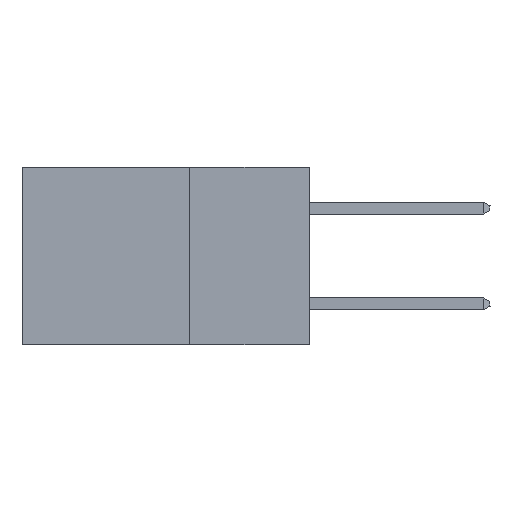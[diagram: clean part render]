
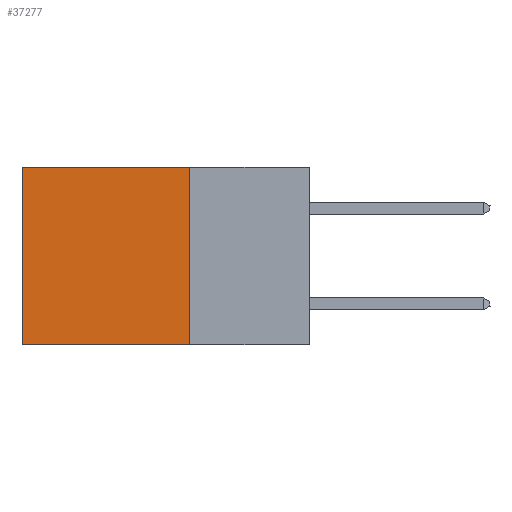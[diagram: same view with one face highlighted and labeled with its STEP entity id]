
A CAD part, left-side view. The second image highlights one B-rep face of the part: STEP entity #37277.
In plain terms, the highlighted planar face has unit normal (-1, 0, 0).
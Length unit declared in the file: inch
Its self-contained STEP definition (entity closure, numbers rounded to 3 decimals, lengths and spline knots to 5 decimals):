
#478 = VECTOR ( 'NONE', #3477, 39.37008 ) ;
#698 = DIRECTION ( 'NONE',  ( 0., 0., -1. ) ) ;
#1804 = VERTEX_POINT ( 'NONE', #7959 ) ;
#3477 = DIRECTION ( 'NONE',  ( 0., 0., -1. ) ) ;
#5650 = LINE ( 'NONE', #15733, #6616 ) ;
#5654 = CARTESIAN_POINT ( 'NONE',  ( 0.2875, 0.6, 0. ) ) ;
#6616 = VECTOR ( 'NONE', #9685, 39.37008 ) ;
#7645 = VECTOR ( 'NONE', #698, 39.37008 ) ;
#7959 = CARTESIAN_POINT ( 'NONE',  ( 0.2875, 0.25, -0.37 ) ) ;
#8752 = LINE ( 'NONE', #30887, #478 ) ;
#8834 = CARTESIAN_POINT ( 'NONE',  ( 0.2875, 0.6, -0.37 ) ) ;
#8905 = ORIENTED_EDGE ( 'NONE', *, *, #13573, .F. ) ;
#9685 = DIRECTION ( 'NONE',  ( 0., 1., 0. ) ) ;
#10686 = ORIENTED_EDGE ( 'NONE', *, *, #37093, .F. ) ;
#11004 = EDGE_CURVE ( 'NONE', #24900, #12206, #8752, .T. ) ;
#12206 = VERTEX_POINT ( 'NONE', #8834 ) ;
#12350 = VECTOR ( 'NONE', #13617, 39.37008 ) ;
#13573 = EDGE_CURVE ( 'NONE', #31010, #1804, #31904, .T. ) ;
#13617 = DIRECTION ( 'NONE',  ( 0., 1., 0. ) ) ;
#14423 = PLANE ( 'NONE',  #36116 ) ;
#15595 = EDGE_CURVE ( 'NONE', #31010, #24900, #5650, .T. ) ;
#15733 = CARTESIAN_POINT ( 'NONE',  ( 0.2875, 0.25, 0. ) ) ;
#16137 = CARTESIAN_POINT ( 'NONE',  ( 0.2875, 0.25, 0. ) ) ;
#20641 = DIRECTION ( 'NONE',  ( 0., 0., -1. ) ) ;
#21948 = FACE_OUTER_BOUND ( 'NONE', #30113, .T. ) ;
#23592 = CARTESIAN_POINT ( 'NONE',  ( 0.2875, 0.25, 0. ) ) ;
#24900 = VERTEX_POINT ( 'NONE', #5654 ) ;
#26756 = ORIENTED_EDGE ( 'NONE', *, *, #11004, .T. ) ;
#28531 = LINE ( 'NONE', #28797, #12350 ) ;
#28797 = CARTESIAN_POINT ( 'NONE',  ( 0.2875, 0.25, -0.37 ) ) ;
#30113 = EDGE_LOOP ( 'NONE', ( #26756, #10686, #8905, #38354 ) ) ;
#30887 = CARTESIAN_POINT ( 'NONE',  ( 0.2875, 0.6, 0. ) ) ;
#31010 = VERTEX_POINT ( 'NONE', #23592 ) ;
#31904 = LINE ( 'NONE', #16137, #7645 ) ;
#35623 = CARTESIAN_POINT ( 'NONE',  ( 0.2875, 0.25, 0. ) ) ;
#36116 = AXIS2_PLACEMENT_3D ( 'NONE', #35623, #38633, #20641 ) ;
#37093 = EDGE_CURVE ( 'NONE', #1804, #12206, #28531, .T. ) ;
#37277 = ADVANCED_FACE ( 'NONE', ( #21948 ), #14423, .F. ) ;
#38354 = ORIENTED_EDGE ( 'NONE', *, *, #15595, .T. ) ;
#38633 = DIRECTION ( 'NONE',  ( 1., 0., 0. ) ) ;
